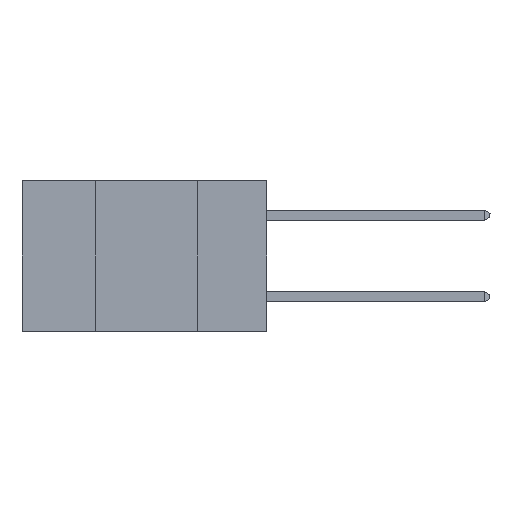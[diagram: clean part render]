
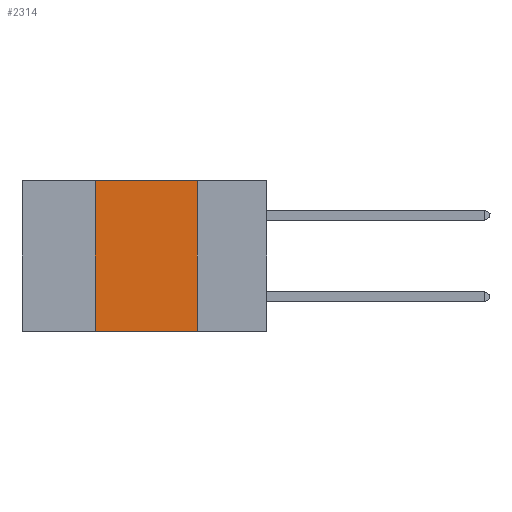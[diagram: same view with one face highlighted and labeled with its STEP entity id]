
A CAD part, left-side view. The second image highlights one B-rep face of the part: STEP entity #2314.
In plain terms, the highlighted planar face has unit normal (-1, 0, 0).
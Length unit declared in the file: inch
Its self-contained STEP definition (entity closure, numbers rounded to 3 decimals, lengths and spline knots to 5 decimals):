
#123 = VECTOR ( 'NONE', #24097, 39.37008 ) ;
#2057 = VECTOR ( 'NONE', #17478, 39.37008 ) ;
#2139 = VERTEX_POINT ( 'NONE', #18749 ) ;
#2314 = ADVANCED_FACE ( 'NONE', ( #19082 ), #22313, .F. ) ;
#2797 = CARTESIAN_POINT ( 'NONE',  ( 0., 0.42, 0. ) ) ;
#2804 = EDGE_LOOP ( 'NONE', ( #3042, #28015, #29152, #3324 ) ) ;
#3042 = ORIENTED_EDGE ( 'NONE', *, *, #11135, .F. ) ;
#3324 = ORIENTED_EDGE ( 'NONE', *, *, #18522, .T. ) ;
#8652 = DIRECTION ( 'NONE',  ( 0., -1., 0. ) ) ;
#9379 = DIRECTION ( 'NONE',  ( 1., 0., 0. ) ) ;
#9570 = VECTOR ( 'NONE', #13149, 39.37008 ) ;
#11135 = EDGE_CURVE ( 'NONE', #2139, #13709, #14907, .T. ) ;
#11512 = LINE ( 'NONE', #26463, #123 ) ;
#13077 = AXIS2_PLACEMENT_3D ( 'NONE', #32647, #9379, #30109 ) ;
#13149 = DIRECTION ( 'NONE',  ( 0., 0., 1. ) ) ;
#13709 = VERTEX_POINT ( 'NONE', #28391 ) ;
#14249 = CARTESIAN_POINT ( 'NONE',  ( 0., 0.6, -0.37 ) ) ;
#14907 = LINE ( 'NONE', #25420, #2057 ) ;
#15865 = EDGE_CURVE ( 'NONE', #20274, #2139, #11512, .T. ) ;
#17478 = DIRECTION ( 'NONE',  ( 0., 0., -1. ) ) ;
#17713 = CARTESIAN_POINT ( 'NONE',  ( 0., 0.42, 0. ) ) ;
#18522 = EDGE_CURVE ( 'NONE', #31861, #13709, #29368, .T. ) ;
#18749 = CARTESIAN_POINT ( 'NONE',  ( 0., 0.17, 0. ) ) ;
#19082 = FACE_OUTER_BOUND ( 'NONE', #2804, .T. ) ;
#20274 = VERTEX_POINT ( 'NONE', #17713 ) ;
#21237 = EDGE_CURVE ( 'NONE', #31861, #20274, #26057, .T. ) ;
#22313 = PLANE ( 'NONE',  #13077 ) ;
#24097 = DIRECTION ( 'NONE',  ( 0., -1., 0. ) ) ;
#24591 = VECTOR ( 'NONE', #8652, 39.37008 ) ;
#25420 = CARTESIAN_POINT ( 'NONE',  ( 0., 0.17, 0. ) ) ;
#26057 = LINE ( 'NONE', #2797, #9570 ) ;
#26463 = CARTESIAN_POINT ( 'NONE',  ( 0., 0.6, 0. ) ) ;
#28015 = ORIENTED_EDGE ( 'NONE', *, *, #15865, .F. ) ;
#28391 = CARTESIAN_POINT ( 'NONE',  ( 0., 0.17, -0.37 ) ) ;
#29152 = ORIENTED_EDGE ( 'NONE', *, *, #21237, .F. ) ;
#29368 = LINE ( 'NONE', #14249, #24591 ) ;
#30109 = DIRECTION ( 'NONE',  ( 0., 0., -1. ) ) ;
#31085 = CARTESIAN_POINT ( 'NONE',  ( 0., 0.42, -0.37 ) ) ;
#31861 = VERTEX_POINT ( 'NONE', #31085 ) ;
#32647 = CARTESIAN_POINT ( 'NONE',  ( 0., 0.6, 0. ) ) ;
